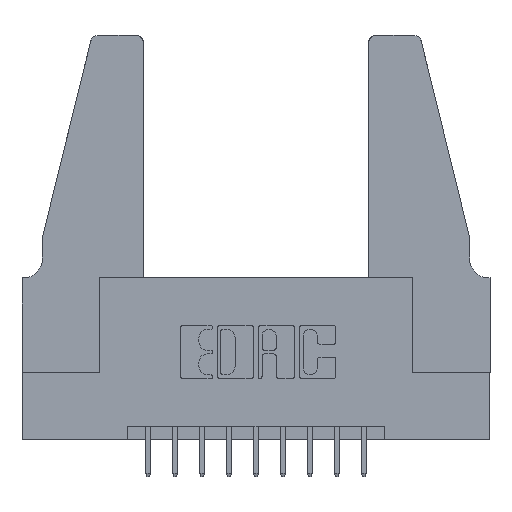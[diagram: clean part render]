
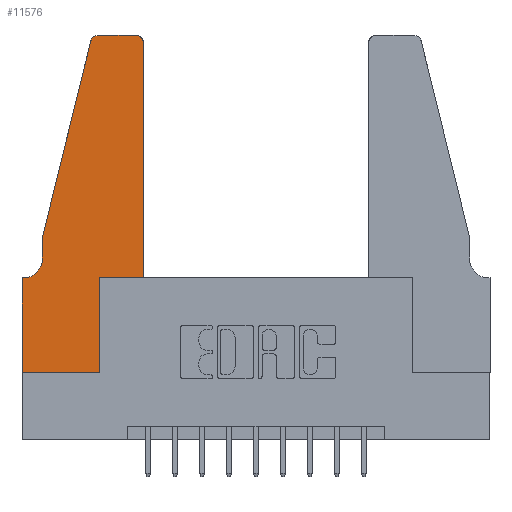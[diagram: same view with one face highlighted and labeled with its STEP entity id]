
A CAD part, top view. The second image highlights one B-rep face of the part: STEP entity #11576.
In plain terms, the highlighted planar face has unit normal (0, 0, 1).
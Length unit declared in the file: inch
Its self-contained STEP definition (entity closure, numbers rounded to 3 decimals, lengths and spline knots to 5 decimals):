
#73 = DIRECTION ( 'NONE',  ( -1., 0., 0. ) ) ;
#140 = DIRECTION ( 'NONE',  ( 0., 0., -1. ) ) ;
#167 = CARTESIAN_POINT ( 'NONE',  ( 0.284, 1.22, 0.37 ) ) ;
#238 = FACE_OUTER_BOUND ( 'NONE', #1390, .T. ) ;
#470 = CIRCLE ( 'NONE', #3987, 0.03 ) ;
#599 = DIRECTION ( 'NONE',  ( 0., 1., 0. ) ) ;
#1042 = CARTESIAN_POINT ( 'NONE',  ( 0., 0.35, 0.37 ) ) ;
#1096 = VERTEX_POINT ( 'NONE', #3021 ) ;
#1126 = AXIS2_PLACEMENT_3D ( 'NONE', #11801, #140, #73 ) ;
#1157 = VECTOR ( 'NONE', #599, 39.37008 ) ;
#1194 = DIRECTION ( 'NONE',  ( 0., 0., 1. ) ) ;
#1340 = DIRECTION ( 'NONE',  ( 1., 0., 0. ) ) ;
#1390 = EDGE_LOOP ( 'NONE', ( #7599, #10274, #6625, #3465, #8513, #2857, #6619, #11379, #7306, #4127, #9893, #9967 ) ) ;
#1412 = DIRECTION ( 'NONE',  ( 1., 0., 0. ) ) ;
#1502 = VERTEX_POINT ( 'NONE', #4202 ) ;
#1562 = VECTOR ( 'NONE', #4277, 39.37008 ) ;
#1576 = EDGE_CURVE ( 'NONE', #5353, #11812, #5045, .T. ) ;
#1689 = CARTESIAN_POINT ( 'NONE',  ( 0., 0.35, 0.37 ) ) ;
#1797 = CARTESIAN_POINT ( 'NONE',  ( 0.4505, 0.35, 0.37 ) ) ;
#1936 = DIRECTION ( 'NONE',  ( 1., 0., 0. ) ) ;
#2125 = VECTOR ( 'NONE', #11806, 39.37008 ) ;
#2152 = CARTESIAN_POINT ( 'NONE',  ( 0.2605, 1.25, 0.37 ) ) ;
#2210 = LINE ( 'NONE', #2152, #1562 ) ;
#2312 = VERTEX_POINT ( 'NONE', #4120 ) ;
#2479 = EDGE_CURVE ( 'NONE', #6351, #4170, #9631, .T. ) ;
#2803 = CARTESIAN_POINT ( 'NONE',  ( 0.0055, 0.35, 0.37 ) ) ;
#2857 = ORIENTED_EDGE ( 'NONE', *, *, #2479, .T. ) ;
#3021 = CARTESIAN_POINT ( 'NONE',  ( 0., 0., 0.37 ) ) ;
#3465 = ORIENTED_EDGE ( 'NONE', *, *, #7970, .T. ) ;
#3704 = CARTESIAN_POINT ( 'NONE',  ( 0.4505, 0.35, 0.37 ) ) ;
#3829 = VERTEX_POINT ( 'NONE', #5220 ) ;
#3970 = VERTEX_POINT ( 'NONE', #9719 ) ;
#3987 = AXIS2_PLACEMENT_3D ( 'NONE', #9849, #8802, #7760 ) ;
#4003 = VERTEX_POINT ( 'NONE', #8695 ) ;
#4120 = CARTESIAN_POINT ( 'NONE',  ( 0.284, 1.25, 0.37 ) ) ;
#4127 = ORIENTED_EDGE ( 'NONE', *, *, #1576, .T. ) ;
#4170 = VERTEX_POINT ( 'NONE', #1689 ) ;
#4202 = CARTESIAN_POINT ( 'NONE',  ( 0.25487, 1.22718, 0.37 ) ) ;
#4277 = DIRECTION ( 'NONE',  ( -1., 0., 0. ) ) ;
#4346 = LINE ( 'NONE', #12843, #2125 ) ;
#4367 = DIRECTION ( 'NONE',  ( 0., 0., 1. ) ) ;
#4613 = EDGE_CURVE ( 'NONE', #4170, #1096, #12496, .T. ) ;
#4760 = EDGE_CURVE ( 'NONE', #3970, #3829, #470, .T. ) ;
#4886 = CIRCLE ( 'NONE', #1126, 0.07 ) ;
#4968 = LINE ( 'NONE', #11638, #6696 ) ;
#5045 = LINE ( 'NONE', #1797, #9508 ) ;
#5197 = CARTESIAN_POINT ( 'NONE',  ( 0., 0., 0.37 ) ) ;
#5220 = CARTESIAN_POINT ( 'NONE',  ( 0.4205, 1.25, 0.37 ) ) ;
#5235 = DIRECTION ( 'NONE',  ( -0.239, -0.971, 0. ) ) ;
#5353 = VERTEX_POINT ( 'NONE', #6601 ) ;
#5563 = LINE ( 'NONE', #9933, #6726 ) ;
#5761 = AXIS2_PLACEMENT_3D ( 'NONE', #1042, #1194, #1340 ) ;
#6173 = DIRECTION ( 'NONE',  ( 1., 0., 0. ) ) ;
#6338 = EDGE_CURVE ( 'NONE', #12327, #5353, #4346, .T. ) ;
#6351 = VERTEX_POINT ( 'NONE', #2803 ) ;
#6467 = EDGE_CURVE ( 'NONE', #1096, #12327, #13338, .T. ) ;
#6601 = CARTESIAN_POINT ( 'NONE',  ( 0.2865, 0.35, 0.37 ) ) ;
#6619 = ORIENTED_EDGE ( 'NONE', *, *, #4613, .T. ) ;
#6625 = ORIENTED_EDGE ( 'NONE', *, *, #10411, .T. ) ;
#6696 = VECTOR ( 'NONE', #5235, 39.37008 ) ;
#6726 = VECTOR ( 'NONE', #9020, 39.37008 ) ;
#6902 = VECTOR ( 'NONE', #12423, 39.37008 ) ;
#6928 = CIRCLE ( 'NONE', #9134, 0.03 ) ;
#7220 = VECTOR ( 'NONE', #1936, 39.37008 ) ;
#7306 = ORIENTED_EDGE ( 'NONE', *, *, #6338, .T. ) ;
#7599 = ORIENTED_EDGE ( 'NONE', *, *, #10049, .T. ) ;
#7656 = PLANE ( 'NONE',  #5761 ) ;
#7681 = CARTESIAN_POINT ( 'NONE',  ( 0.0755, 0.42, 0.37 ) ) ;
#7760 = DIRECTION ( 'NONE',  ( 1., 0., 0. ) ) ;
#7970 = EDGE_CURVE ( 'NONE', #4003, #10651, #5563, .T. ) ;
#8314 = CARTESIAN_POINT ( 'NONE',  ( 0.4505, 0.35, 0.37 ) ) ;
#8513 = ORIENTED_EDGE ( 'NONE', *, *, #10037, .T. ) ;
#8695 = CARTESIAN_POINT ( 'NONE',  ( 0.0755, 0.5, 0.37 ) ) ;
#8802 = DIRECTION ( 'NONE',  ( 0., 0., 1. ) ) ;
#9020 = DIRECTION ( 'NONE',  ( 0., -1., 0. ) ) ;
#9134 = AXIS2_PLACEMENT_3D ( 'NONE', #167, #4367, #1412 ) ;
#9402 = CARTESIAN_POINT ( 'NONE',  ( 0.2865, 0., 0.37 ) ) ;
#9508 = VECTOR ( 'NONE', #6173, 39.37008 ) ;
#9631 = LINE ( 'NONE', #10970, #13319 ) ;
#9719 = CARTESIAN_POINT ( 'NONE',  ( 0.4505, 1.22, 0.37 ) ) ;
#9849 = CARTESIAN_POINT ( 'NONE',  ( 0.4205, 1.22, 0.37 ) ) ;
#9893 = ORIENTED_EDGE ( 'NONE', *, *, #13359, .T. ) ;
#9933 = CARTESIAN_POINT ( 'NONE',  ( 0.0755, 0.5, 0.37 ) ) ;
#9967 = ORIENTED_EDGE ( 'NONE', *, *, #4760, .T. ) ;
#10037 = EDGE_CURVE ( 'NONE', #10651, #6351, #4886, .T. ) ;
#10049 = EDGE_CURVE ( 'NONE', #3829, #2312, #2210, .T. ) ;
#10131 = LINE ( 'NONE', #3704, #1157 ) ;
#10193 = CARTESIAN_POINT ( 'NONE',  ( 0., 0., 0.37 ) ) ;
#10274 = ORIENTED_EDGE ( 'NONE', *, *, #12943, .T. ) ;
#10411 = EDGE_CURVE ( 'NONE', #1502, #4003, #4968, .T. ) ;
#10651 = VERTEX_POINT ( 'NONE', #7681 ) ;
#10772 = DIRECTION ( 'NONE',  ( -1., 0., 0. ) ) ;
#10970 = CARTESIAN_POINT ( 'NONE',  ( 0.0755, 0.35, 0.37 ) ) ;
#11379 = ORIENTED_EDGE ( 'NONE', *, *, #6467, .T. ) ;
#11576 = ADVANCED_FACE ( 'NONE', ( #238 ), #7656, .T. ) ;
#11638 = CARTESIAN_POINT ( 'NONE',  ( 0.0755, 0.5, 0.37 ) ) ;
#11801 = CARTESIAN_POINT ( 'NONE',  ( 0.0055, 0.42, 0.37 ) ) ;
#11806 = DIRECTION ( 'NONE',  ( 0., 1., 0. ) ) ;
#11812 = VERTEX_POINT ( 'NONE', #8314 ) ;
#12327 = VERTEX_POINT ( 'NONE', #9402 ) ;
#12423 = DIRECTION ( 'NONE',  ( 0., -1., 0. ) ) ;
#12496 = LINE ( 'NONE', #5197, #6902 ) ;
#12843 = CARTESIAN_POINT ( 'NONE',  ( 0.2865, 0.35, 0.37 ) ) ;
#12943 = EDGE_CURVE ( 'NONE', #2312, #1502, #6928, .T. ) ;
#13319 = VECTOR ( 'NONE', #10772, 39.37008 ) ;
#13338 = LINE ( 'NONE', #10193, #7220 ) ;
#13359 = EDGE_CURVE ( 'NONE', #11812, #3970, #10131, .T. ) ;
